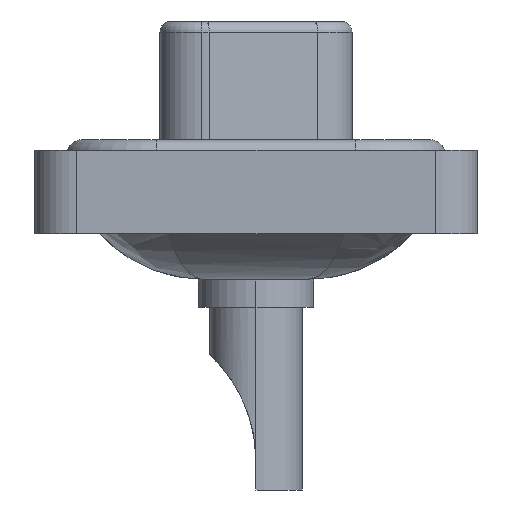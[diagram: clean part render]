
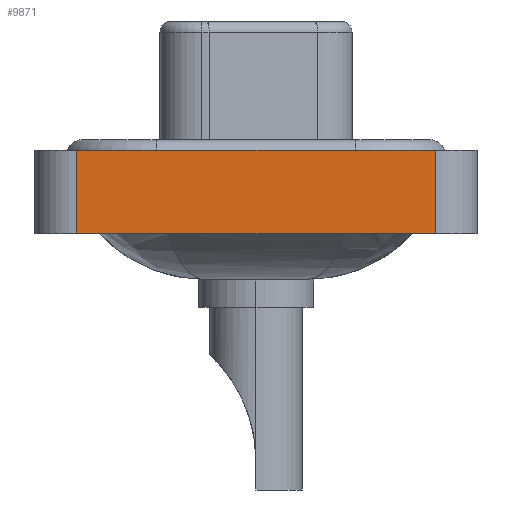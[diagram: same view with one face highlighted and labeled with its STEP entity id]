
A CAD part, left-side view. The second image highlights one B-rep face of the part: STEP entity #9871.
In plain terms, the highlighted planar face has unit normal (-1, 0, 0).
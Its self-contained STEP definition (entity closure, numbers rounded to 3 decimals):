
#496 = VERTEX_POINT ( 'NONE', #6625 ) ;
#601 = CARTESIAN_POINT ( 'NONE',  ( -7.35, 8.55, 0.4 ) ) ;
#824 = CARTESIAN_POINT ( 'NONE',  ( -7.35, -8.55, -3.6 ) ) ;
#1621 = EDGE_CURVE ( 'NONE', #14895, #11547, #11295, .T. ) ;
#2388 = CARTESIAN_POINT ( 'NONE',  ( -7.35, -8.55, -3.6 ) ) ;
#2489 = DIRECTION ( 'NONE',  ( 0., 0., 1. ) ) ;
#3154 = EDGE_CURVE ( 'NONE', #14895, #6598, #12630, .T. ) ;
#4055 = VECTOR ( 'NONE', #5578, 1000. ) ;
#4323 = AXIS2_PLACEMENT_3D ( 'NONE', #2388, #8064, #18203 ) ;
#5578 = DIRECTION ( 'NONE',  ( 0., -1., 0. ) ) ;
#6070 = DIRECTION ( 'NONE',  ( 0., 0., 1. ) ) ;
#6598 = VERTEX_POINT ( 'NONE', #12813 ) ;
#6625 = CARTESIAN_POINT ( 'NONE',  ( -7.35, -8.55, 0.4 ) ) ;
#6749 = ORIENTED_EDGE ( 'NONE', *, *, #1621, .F. ) ;
#6838 = FACE_OUTER_BOUND ( 'NONE', #8313, .T. ) ;
#7402 = VECTOR ( 'NONE', #2489, 1000. ) ;
#8064 = DIRECTION ( 'NONE',  ( -1., 0., 0. ) ) ;
#8069 = CARTESIAN_POINT ( 'NONE',  ( -7.35, -8.55, -3.6 ) ) ;
#8076 = LINE ( 'NONE', #824, #7402 ) ;
#8251 = PLANE ( 'NONE',  #4323 ) ;
#8313 = EDGE_LOOP ( 'NONE', ( #9388, #12614, #6749, #8957 ) ) ;
#8957 = ORIENTED_EDGE ( 'NONE', *, *, #3154, .T. ) ;
#9388 = ORIENTED_EDGE ( 'NONE', *, *, #17390, .T. ) ;
#9871 = ADVANCED_FACE ( 'NONE', ( #6838 ), #8251, .T. ) ;
#10086 = CARTESIAN_POINT ( 'NONE',  ( -7.35, 8.55, -3.6 ) ) ;
#10166 = CARTESIAN_POINT ( 'NONE',  ( -7.35, 8.55, -3.6 ) ) ;
#10645 = VECTOR ( 'NONE', #6070, 1000. ) ;
#11295 = LINE ( 'NONE', #10086, #10645 ) ;
#11415 = EDGE_CURVE ( 'NONE', #11547, #496, #16936, .T. ) ;
#11547 = VERTEX_POINT ( 'NONE', #601 ) ;
#12614 = ORIENTED_EDGE ( 'NONE', *, *, #11415, .F. ) ;
#12630 = LINE ( 'NONE', #8069, #13231 ) ;
#12813 = CARTESIAN_POINT ( 'NONE',  ( -7.35, -8.55, -3.6 ) ) ;
#13231 = VECTOR ( 'NONE', #18300, 1000. ) ;
#14049 = CARTESIAN_POINT ( 'NONE',  ( -7.35, -8.55, 0.4 ) ) ;
#14895 = VERTEX_POINT ( 'NONE', #10166 ) ;
#16936 = LINE ( 'NONE', #14049, #4055 ) ;
#17390 = EDGE_CURVE ( 'NONE', #6598, #496, #8076, .T. ) ;
#18203 = DIRECTION ( 'NONE',  ( 0., 0., 1. ) ) ;
#18300 = DIRECTION ( 'NONE',  ( 0., -1., 0. ) ) ;
